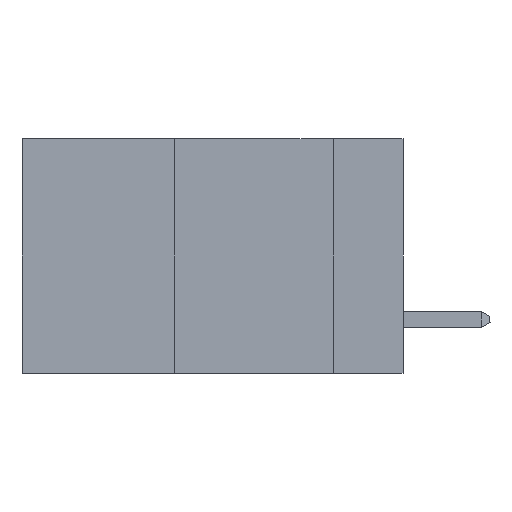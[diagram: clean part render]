
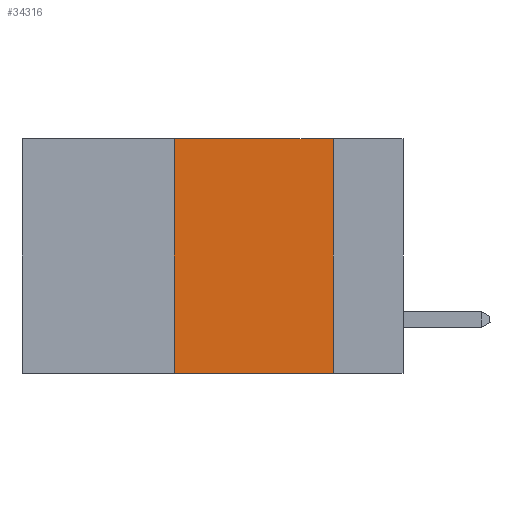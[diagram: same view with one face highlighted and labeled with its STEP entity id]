
A CAD part, left-side view. The second image highlights one B-rep face of the part: STEP entity #34316.
In plain terms, the highlighted planar face has unit normal (-1, 0, 0).
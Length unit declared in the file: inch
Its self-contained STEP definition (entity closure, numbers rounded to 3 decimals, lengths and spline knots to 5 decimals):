
#239 = ORIENTED_EDGE ( 'NONE', *, *, #33177, .F. ) ;
#794 = ORIENTED_EDGE ( 'NONE', *, *, #5178, .F. ) ;
#1737 = VERTEX_POINT ( 'NONE', #14385 ) ;
#1913 = FACE_OUTER_BOUND ( 'NONE', #11925, .T. ) ;
#1930 = DIRECTION ( 'NONE',  ( 1., 0., 0. ) ) ;
#1988 = CARTESIAN_POINT ( 'NONE',  ( 0., 0.6, -0.37 ) ) ;
#3099 = VERTEX_POINT ( 'NONE', #13891 ) ;
#3780 = CARTESIAN_POINT ( 'NONE',  ( 0., 0.36, 0. ) ) ;
#4903 = CARTESIAN_POINT ( 'NONE',  ( 0., 0.36, 0. ) ) ;
#5178 = EDGE_CURVE ( 'NONE', #3099, #35303, #31507, .T. ) ;
#9340 = DIRECTION ( 'NONE',  ( 0., -1., 0. ) ) ;
#9619 = EDGE_CURVE ( 'NONE', #3099, #1737, #19853, .T. ) ;
#11070 = CARTESIAN_POINT ( 'NONE',  ( 0., 0.11, 0. ) ) ;
#11925 = EDGE_LOOP ( 'NONE', ( #39276, #239, #794, #29461 ) ) ;
#12145 = DIRECTION ( 'NONE',  ( 0., 0., -1. ) ) ;
#13891 = CARTESIAN_POINT ( 'NONE',  ( 0., 0.36, -0.37 ) ) ;
#14385 = CARTESIAN_POINT ( 'NONE',  ( 0., 0.11, -0.37 ) ) ;
#15476 = PLANE ( 'NONE',  #21144 ) ;
#17418 = CARTESIAN_POINT ( 'NONE',  ( 0., 0.11, 0. ) ) ;
#17556 = VECTOR ( 'NONE', #18201, 39.37008 ) ;
#17621 = DIRECTION ( 'NONE',  ( 0., 0., -1. ) ) ;
#18201 = DIRECTION ( 'NONE',  ( 0., 0., 1. ) ) ;
#18960 = CARTESIAN_POINT ( 'NONE',  ( 0., 0.6, 0. ) ) ;
#19853 = LINE ( 'NONE', #1988, #31154 ) ;
#21144 = AXIS2_PLACEMENT_3D ( 'NONE', #18960, #1930, #12145 ) ;
#24220 = LINE ( 'NONE', #11070, #40385 ) ;
#29461 = ORIENTED_EDGE ( 'NONE', *, *, #9619, .T. ) ;
#30774 = LINE ( 'NONE', #37319, #42075 ) ;
#31154 = VECTOR ( 'NONE', #9340, 39.37008 ) ;
#31507 = LINE ( 'NONE', #3780, #17556 ) ;
#32719 = VERTEX_POINT ( 'NONE', #17418 ) ;
#33177 = EDGE_CURVE ( 'NONE', #35303, #32719, #30774, .T. ) ;
#34131 = EDGE_CURVE ( 'NONE', #32719, #1737, #24220, .T. ) ;
#34316 = ADVANCED_FACE ( 'NONE', ( #1913 ), #15476, .F. ) ;
#35303 = VERTEX_POINT ( 'NONE', #4903 ) ;
#37319 = CARTESIAN_POINT ( 'NONE',  ( 0., 0.6, 0. ) ) ;
#37773 = DIRECTION ( 'NONE',  ( 0., -1., 0. ) ) ;
#39276 = ORIENTED_EDGE ( 'NONE', *, *, #34131, .F. ) ;
#40385 = VECTOR ( 'NONE', #17621, 39.37008 ) ;
#42075 = VECTOR ( 'NONE', #37773, 39.37008 ) ;
